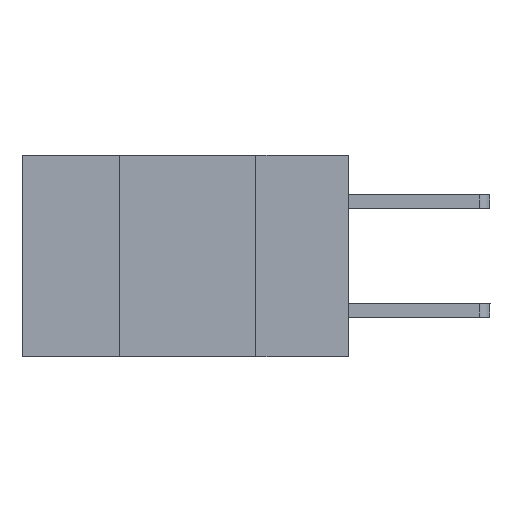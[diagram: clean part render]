
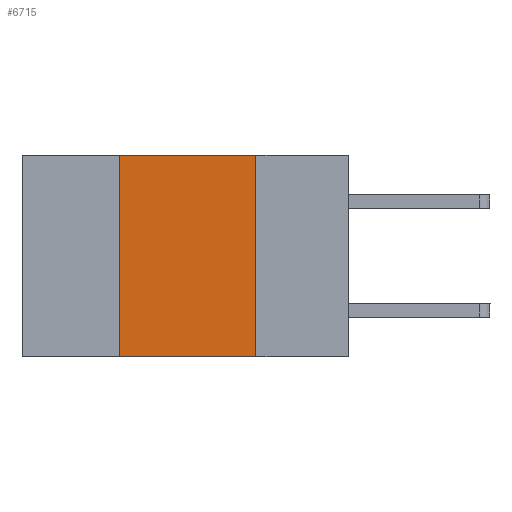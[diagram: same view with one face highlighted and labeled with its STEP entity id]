
A CAD part, left-side view. The second image highlights one B-rep face of the part: STEP entity #6715.
In plain terms, the highlighted planar face has unit normal (-1, 0, 0).
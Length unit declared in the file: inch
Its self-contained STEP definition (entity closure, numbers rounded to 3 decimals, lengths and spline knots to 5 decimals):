
#630 = EDGE_CURVE ( 'NONE', #2955, #6678, #6049, .T. ) ;
#858 = CARTESIAN_POINT ( 'NONE',  ( 0., 0.17, 0. ) ) ;
#1086 = ORIENTED_EDGE ( 'NONE', *, *, #6310, .F. ) ;
#1728 = CARTESIAN_POINT ( 'NONE',  ( 0., 0.17, 0. ) ) ;
#1901 = CARTESIAN_POINT ( 'NONE',  ( 0., 0.17, -0.37 ) ) ;
#2182 = FACE_OUTER_BOUND ( 'NONE', #5552, .T. ) ;
#2291 = ORIENTED_EDGE ( 'NONE', *, *, #2384, .F. ) ;
#2384 = EDGE_CURVE ( 'NONE', #2955, #3798, #6920, .T. ) ;
#2654 = DIRECTION ( 'NONE',  ( 0., 0., -1. ) ) ;
#2955 = VERTEX_POINT ( 'NONE', #7186 ) ;
#3460 = VECTOR ( 'NONE', #4664, 39.37008 ) ;
#3525 = CARTESIAN_POINT ( 'NONE',  ( 0., 0.42, 0. ) ) ;
#3567 = VECTOR ( 'NONE', #8880, 39.37008 ) ;
#3666 = VECTOR ( 'NONE', #4626, 39.37008 ) ;
#3772 = ORIENTED_EDGE ( 'NONE', *, *, #6286, .F. ) ;
#3798 = VERTEX_POINT ( 'NONE', #4296 ) ;
#4219 = LINE ( 'NONE', #4587, #3666 ) ;
#4288 = VECTOR ( 'NONE', #6267, 39.37008 ) ;
#4296 = CARTESIAN_POINT ( 'NONE',  ( 0., 0.42, 0. ) ) ;
#4422 = CARTESIAN_POINT ( 'NONE',  ( 0., 0.6, -0.37 ) ) ;
#4587 = CARTESIAN_POINT ( 'NONE',  ( 0., 0.6, 0. ) ) ;
#4626 = DIRECTION ( 'NONE',  ( 0., -1., 0. ) ) ;
#4664 = DIRECTION ( 'NONE',  ( 0., 0., -1. ) ) ;
#5245 = LINE ( 'NONE', #1728, #3460 ) ;
#5472 = CARTESIAN_POINT ( 'NONE',  ( 0., 0.6, 0. ) ) ;
#5552 = EDGE_LOOP ( 'NONE', ( #3772, #1086, #2291, #5605 ) ) ;
#5605 = ORIENTED_EDGE ( 'NONE', *, *, #630, .T. ) ;
#6049 = LINE ( 'NONE', #4422, #3567 ) ;
#6267 = DIRECTION ( 'NONE',  ( 0., 0., 1. ) ) ;
#6286 = EDGE_CURVE ( 'NONE', #7941, #6678, #5245, .T. ) ;
#6310 = EDGE_CURVE ( 'NONE', #3798, #7941, #4219, .T. ) ;
#6678 = VERTEX_POINT ( 'NONE', #1901 ) ;
#6715 = ADVANCED_FACE ( 'NONE', ( #2182 ), #7050, .F. ) ;
#6920 = LINE ( 'NONE', #3525, #4288 ) ;
#6986 = DIRECTION ( 'NONE',  ( 1., 0., 0. ) ) ;
#7050 = PLANE ( 'NONE',  #7827 ) ;
#7186 = CARTESIAN_POINT ( 'NONE',  ( 0., 0.42, -0.37 ) ) ;
#7827 = AXIS2_PLACEMENT_3D ( 'NONE', #5472, #6986, #2654 ) ;
#7941 = VERTEX_POINT ( 'NONE', #858 ) ;
#8880 = DIRECTION ( 'NONE',  ( 0., -1., 0. ) ) ;
